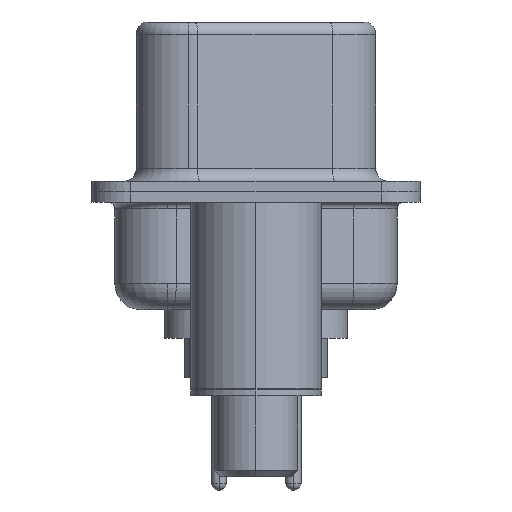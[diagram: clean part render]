
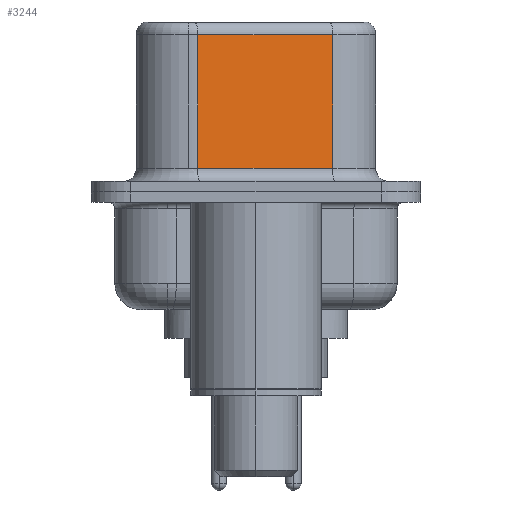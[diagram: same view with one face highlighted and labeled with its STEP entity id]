
A CAD part, left-side view. The second image highlights one B-rep face of the part: STEP entity #3244.
In plain terms, the highlighted planar face has unit normal (-0.985, -0.174, 0).
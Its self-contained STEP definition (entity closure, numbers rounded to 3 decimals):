
#1585 = VERTEX_POINT ( 'NONE', #20327 ) ;
#2431 = DIRECTION ( 'NONE',  ( -0.174, 0.985, 0. ) ) ;
#2518 = VERTEX_POINT ( 'NONE', #11238 ) ;
#3244 = ADVANCED_FACE ( 'NONE', ( #14211 ), #3580, .F. ) ;
#3580 = PLANE ( 'NONE',  #7434 ) ;
#3799 = CARTESIAN_POINT ( 'NONE',  ( 4.585, -2.927, 6.52 ) ) ;
#4052 = EDGE_CURVE ( 'NONE', #2518, #1585, #15974, .T. ) ;
#5004 = CARTESIAN_POINT ( 'NONE',  ( 3.675, 2.233, 0.9 ) ) ;
#5552 = EDGE_CURVE ( 'NONE', #12228, #1585, #10551, .T. ) ;
#5653 = EDGE_CURVE ( 'NONE', #14588, #12228, #18307, .T. ) ;
#6050 = DIRECTION ( 'NONE',  ( 0., 0., -1. ) ) ;
#6947 = DIRECTION ( 'NONE',  ( -0.174, 0.985, 0. ) ) ;
#7434 = AXIS2_PLACEMENT_3D ( 'NONE', #3799, #19734, #6947 ) ;
#7785 = CARTESIAN_POINT ( 'NONE',  ( 4.585, -2.927, 6.52 ) ) ;
#7985 = EDGE_LOOP ( 'NONE', ( #18242, #14582, #18758, #8537 ) ) ;
#8537 = ORIENTED_EDGE ( 'NONE', *, *, #5552, .T. ) ;
#8622 = DIRECTION ( 'NONE',  ( 0.174, -0.985, 0. ) ) ;
#9012 = VECTOR ( 'NONE', #16272, 1000. ) ;
#10134 = CARTESIAN_POINT ( 'NONE',  ( 4.585, -2.927, 0.9 ) ) ;
#10551 = LINE ( 'NONE', #10134, #18820 ) ;
#11070 = VECTOR ( 'NONE', #6050, 1000. ) ;
#11128 = EDGE_CURVE ( 'NONE', #2518, #14588, #14170, .T. ) ;
#11238 = CARTESIAN_POINT ( 'NONE',  ( 4.585, -2.927, 6.02 ) ) ;
#12228 = VERTEX_POINT ( 'NONE', #5004 ) ;
#14170 = LINE ( 'NONE', #20444, #18044 ) ;
#14211 = FACE_OUTER_BOUND ( 'NONE', #7985, .T. ) ;
#14582 = ORIENTED_EDGE ( 'NONE', *, *, #11128, .T. ) ;
#14588 = VERTEX_POINT ( 'NONE', #20138 ) ;
#15295 = CARTESIAN_POINT ( 'NONE',  ( 3.675, 2.233, 6.52 ) ) ;
#15974 = LINE ( 'NONE', #7785, #11070 ) ;
#16272 = DIRECTION ( 'NONE',  ( 0., 0., -1. ) ) ;
#18044 = VECTOR ( 'NONE', #2431, 1000. ) ;
#18242 = ORIENTED_EDGE ( 'NONE', *, *, #4052, .F. ) ;
#18307 = LINE ( 'NONE', #15295, #9012 ) ;
#18758 = ORIENTED_EDGE ( 'NONE', *, *, #5653, .T. ) ;
#18820 = VECTOR ( 'NONE', #8622, 1000. ) ;
#19734 = DIRECTION ( 'NONE',  ( 0.985, 0.174, 0. ) ) ;
#20138 = CARTESIAN_POINT ( 'NONE',  ( 3.675, 2.233, 6.02 ) ) ;
#20327 = CARTESIAN_POINT ( 'NONE',  ( 4.585, -2.927, 0.9 ) ) ;
#20444 = CARTESIAN_POINT ( 'NONE',  ( 4.585, -2.927, 6.02 ) ) ;
